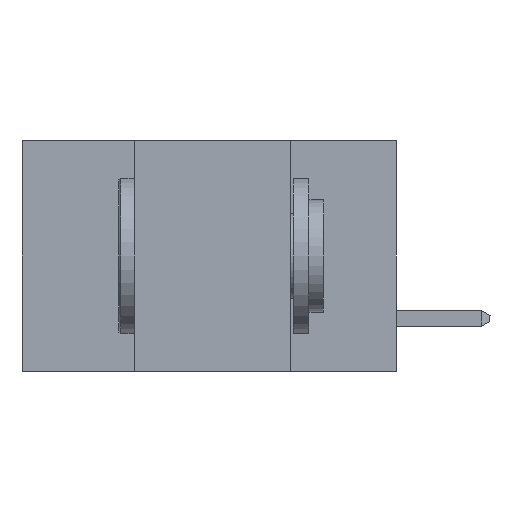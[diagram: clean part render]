
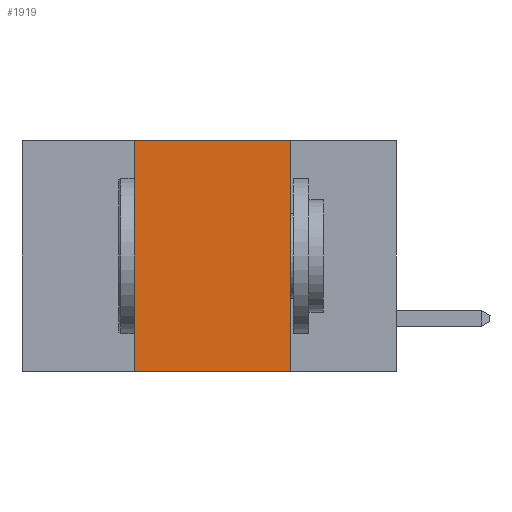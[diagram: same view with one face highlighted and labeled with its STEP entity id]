
A CAD part, left-side view. The second image highlights one B-rep face of the part: STEP entity #1919.
In plain terms, the highlighted planar face has unit normal (-1, 0, 0).
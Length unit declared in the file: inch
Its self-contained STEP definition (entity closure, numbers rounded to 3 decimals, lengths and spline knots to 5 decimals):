
#161 = CARTESIAN_POINT ( 'NONE',  ( 0., 0.6, 0. ) ) ;
#441 = VECTOR ( 'NONE', #22515, 39.37008 ) ;
#954 = VECTOR ( 'NONE', #10152, 39.37008 ) ;
#1252 = CARTESIAN_POINT ( 'NONE',  ( 0., 0.17, -0.37 ) ) ;
#1610 = LINE ( 'NONE', #20499, #22412 ) ;
#1919 = ADVANCED_FACE ( 'NONE', ( #4285 ), #20621, .F. ) ;
#3054 = EDGE_CURVE ( 'NONE', #21203, #8914, #15873, .T. ) ;
#4285 = FACE_OUTER_BOUND ( 'NONE', #5646, .T. ) ;
#4733 = CARTESIAN_POINT ( 'NONE',  ( 0., 0.42, -0.37 ) ) ;
#5646 = EDGE_LOOP ( 'NONE', ( #14363, #13164, #15181, #10022 ) ) ;
#6153 = DIRECTION ( 'NONE',  ( 0., 0., -1. ) ) ;
#7039 = VECTOR ( 'NONE', #6153, 39.37008 ) ;
#8914 = VERTEX_POINT ( 'NONE', #15752 ) ;
#9534 = EDGE_CURVE ( 'NONE', #8914, #15753, #11782, .T. ) ;
#10022 = ORIENTED_EDGE ( 'NONE', *, *, #10949, .T. ) ;
#10152 = DIRECTION ( 'NONE',  ( 0., 0., 1. ) ) ;
#10204 = DIRECTION ( 'NONE',  ( 0., -1., 0. ) ) ;
#10949 = EDGE_CURVE ( 'NONE', #15556, #15753, #1610, .T. ) ;
#11782 = LINE ( 'NONE', #18747, #7039 ) ;
#11943 = DIRECTION ( 'NONE',  ( 0., 0., -1. ) ) ;
#13164 = ORIENTED_EDGE ( 'NONE', *, *, #3054, .F. ) ;
#14363 = ORIENTED_EDGE ( 'NONE', *, *, #9534, .F. ) ;
#14727 = DIRECTION ( 'NONE',  ( 1., 0., 0. ) ) ;
#15181 = ORIENTED_EDGE ( 'NONE', *, *, #21124, .F. ) ;
#15556 = VERTEX_POINT ( 'NONE', #4733 ) ;
#15752 = CARTESIAN_POINT ( 'NONE',  ( 0., 0.17, 0. ) ) ;
#15753 = VERTEX_POINT ( 'NONE', #1252 ) ;
#15873 = LINE ( 'NONE', #161, #441 ) ;
#16966 = CARTESIAN_POINT ( 'NONE',  ( 0., 0.6, 0. ) ) ;
#18261 = AXIS2_PLACEMENT_3D ( 'NONE', #16966, #14727, #11943 ) ;
#18740 = CARTESIAN_POINT ( 'NONE',  ( 0., 0.42, -0.37 ) ) ;
#18747 = CARTESIAN_POINT ( 'NONE',  ( 0., 0.17, -0.37 ) ) ;
#18959 = CARTESIAN_POINT ( 'NONE',  ( 0., 0.42, 0. ) ) ;
#20454 = LINE ( 'NONE', #18740, #954 ) ;
#20499 = CARTESIAN_POINT ( 'NONE',  ( 0., 0.6, -0.37 ) ) ;
#20621 = PLANE ( 'NONE',  #18261 ) ;
#21124 = EDGE_CURVE ( 'NONE', #15556, #21203, #20454, .T. ) ;
#21203 = VERTEX_POINT ( 'NONE', #18959 ) ;
#22412 = VECTOR ( 'NONE', #10204, 39.37008 ) ;
#22515 = DIRECTION ( 'NONE',  ( 0., -1., 0. ) ) ;
